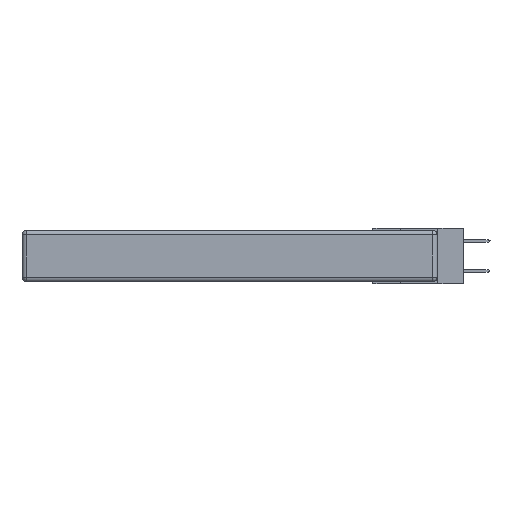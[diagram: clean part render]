
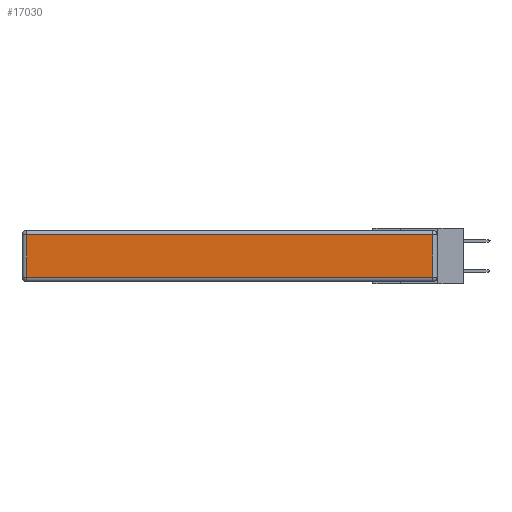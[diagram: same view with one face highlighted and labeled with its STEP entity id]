
A CAD part, left-side view. The second image highlights one B-rep face of the part: STEP entity #17030.
In plain terms, the highlighted planar face has unit normal (-1, 0, 0).
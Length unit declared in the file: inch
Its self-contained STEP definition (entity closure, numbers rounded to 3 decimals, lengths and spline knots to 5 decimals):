
#787 = CARTESIAN_POINT ( 'NONE',  ( 0., 0., -0.343 ) ) ;
#1445 = CARTESIAN_POINT ( 'NONE',  ( 0., 2.75, -0.03 ) ) ;
#1901 = AXIS2_PLACEMENT_3D ( 'NONE', #787, #12495, #5835 ) ;
#3162 = DIRECTION ( 'NONE',  ( 0., 1., 0. ) ) ;
#3427 = DIRECTION ( 'NONE',  ( 0., -1., 0. ) ) ;
#3440 = CARTESIAN_POINT ( 'NONE',  ( 0., 0.03, -0.343 ) ) ;
#4352 = ORIENTED_EDGE ( 'NONE', *, *, #9532, .T. ) ;
#5058 = VECTOR ( 'NONE', #3162, 39.37008 ) ;
#5252 = VECTOR ( 'NONE', #8372, 39.37008 ) ;
#5701 = PLANE ( 'NONE',  #1901 ) ;
#5835 = DIRECTION ( 'NONE',  ( 0., 0., 1. ) ) ;
#6614 = CARTESIAN_POINT ( 'NONE',  ( 0., 0.03, -0.03 ) ) ;
#7420 = VERTEX_POINT ( 'NONE', #19934 ) ;
#8349 = EDGE_CURVE ( 'NONE', #7420, #17594, #15892, .T. ) ;
#8372 = DIRECTION ( 'NONE',  ( 0., 0., 1. ) ) ;
#8405 = EDGE_CURVE ( 'NONE', #20554, #7420, #21761, .T. ) ;
#8463 = DIRECTION ( 'NONE',  ( 0., 0., -1. ) ) ;
#8496 = CARTESIAN_POINT ( 'NONE',  ( 0., 0., -0.313 ) ) ;
#9417 = CARTESIAN_POINT ( 'NONE',  ( 0., 0.03, -0.313 ) ) ;
#9532 = EDGE_CURVE ( 'NONE', #17594, #13870, #11490, .T. ) ;
#9731 = ORIENTED_EDGE ( 'NONE', *, *, #15219, .T. ) ;
#9794 = VECTOR ( 'NONE', #8463, 39.37008 ) ;
#10821 = EDGE_LOOP ( 'NONE', ( #4352, #9731, #21795, #17255 ) ) ;
#11490 = LINE ( 'NONE', #8496, #13863 ) ;
#11602 = LINE ( 'NONE', #3440, #5252 ) ;
#11810 = CARTESIAN_POINT ( 'NONE',  ( 0., 2.72, -0.343 ) ) ;
#12030 = CARTESIAN_POINT ( 'NONE',  ( 0., 2.72, -0.313 ) ) ;
#12495 = DIRECTION ( 'NONE',  ( -1., 0., 0. ) ) ;
#13863 = VECTOR ( 'NONE', #3427, 39.37008 ) ;
#13870 = VERTEX_POINT ( 'NONE', #9417 ) ;
#15219 = EDGE_CURVE ( 'NONE', #13870, #20554, #11602, .T. ) ;
#15892 = LINE ( 'NONE', #11810, #9794 ) ;
#17030 = ADVANCED_FACE ( 'NONE', ( #20469 ), #5701, .T. ) ;
#17255 = ORIENTED_EDGE ( 'NONE', *, *, #8349, .T. ) ;
#17594 = VERTEX_POINT ( 'NONE', #12030 ) ;
#19934 = CARTESIAN_POINT ( 'NONE',  ( 0., 2.72, -0.03 ) ) ;
#20469 = FACE_OUTER_BOUND ( 'NONE', #10821, .T. ) ;
#20554 = VERTEX_POINT ( 'NONE', #6614 ) ;
#21761 = LINE ( 'NONE', #1445, #5058 ) ;
#21795 = ORIENTED_EDGE ( 'NONE', *, *, #8405, .T. ) ;
